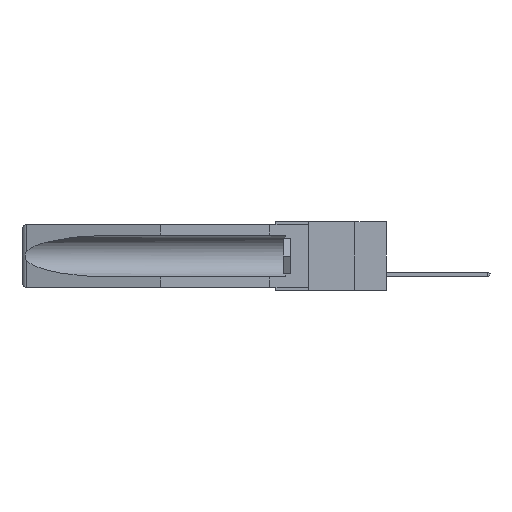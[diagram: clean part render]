
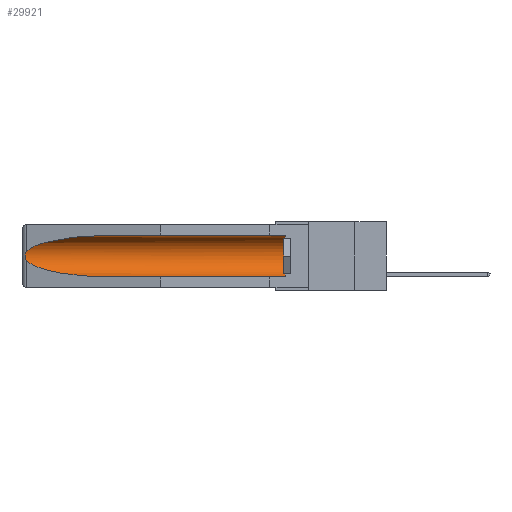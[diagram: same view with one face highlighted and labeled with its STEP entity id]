
A CAD part, left-side view. The second image highlights one B-rep face of the part: STEP entity #29921.
In plain terms, the highlighted cylindrical face has radius 2.857 mm (diameter 5.715 mm), a partial arc.
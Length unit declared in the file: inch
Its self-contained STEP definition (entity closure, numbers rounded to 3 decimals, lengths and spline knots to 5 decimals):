
#278 = EDGE_CURVE ( 'NONE', #11453, #24854, #19707, .T. ) ;
#771 = DIRECTION ( 'NONE',  ( 0., 0., 1. ) ) ;
#850 = CIRCLE ( 'NONE', #26483, 0.1125 ) ;
#1645 = VECTOR ( 'NONE', #17413, 39.37008 ) ;
#2720 = ORIENTED_EDGE ( 'NONE', *, *, #6844, .F. ) ;
#3083 = DIRECTION ( 'NONE',  ( 0., 1., 0. ) ) ;
#3252 = VERTEX_POINT ( 'NONE', #25506 ) ;
#3462 = ORIENTED_EDGE ( 'NONE', *, *, #23596, .T. ) ;
#3466 = CARTESIAN_POINT ( 'NONE',  ( 0.26537, 1.52718, -0.19328 ) ) ;
#4038 = CARTESIAN_POINT ( 'NONE',  ( 0.26597, 1.52961, -0.15275 ) ) ;
#6283 = CARTESIAN_POINT ( 'NONE',  ( 0.26537, 1.52718, -0.14972 ) ) ;
#6343 = ORIENTED_EDGE ( 'NONE', *, *, #21340, .T. ) ;
#6844 = EDGE_CURVE ( 'NONE', #32537, #19119, #28344, .T. ) ;
#7415 = CARTESIAN_POINT ( 'NONE',  ( 0.26654, 1.53092, -0.15636 ) ) ;
#8424 = ORIENTED_EDGE ( 'NONE', *, *, #31454, .T. ) ;
#8873 = CARTESIAN_POINT ( 'NONE',  ( 0.21114, 1.30732, -0.284 ) ) ;
#8904 = B_SPLINE_CURVE_WITH_KNOTS ( 'NONE', 3,
 ( #14223, #4038, #7415, #9836, #14652, #14762, #9950, #12478, #20030, #25083 ),
 .UNSPECIFIED., .F., .F.,
 ( 4, 2, 2, 2, 4 ),
 ( 0., 0.00029, 0.00058, 0.00087, 0.00117 ),
 .UNSPECIFIED. ) ;
#9836 = CARTESIAN_POINT ( 'NONE',  ( 0.2673, 1.5327, -0.16383 ) ) ;
#9950 = CARTESIAN_POINT ( 'NONE',  ( 0.2673, 1.53269, -0.17917 ) ) ;
#10229 = EDGE_CURVE ( 'NONE', #3252, #24516, #8904, .T. ) ;
#11239 = DIRECTION ( 'NONE',  ( 0., 0., 1. ) ) ;
#11369 = CARTESIAN_POINT ( 'NONE',  ( 0.155, 1.07973, -0.059 ) ) ;
#11453 = VERTEX_POINT ( 'NONE', #28151 ) ;
#12120 = ORIENTED_EDGE ( 'NONE', *, *, #278, .T. ) ;
#12140 = CARTESIAN_POINT ( 'NONE',  ( 0.155, 1.07973, -0.284 ) ) ;
#12478 = CARTESIAN_POINT ( 'NONE',  ( 0.26655, 1.53094, -0.18657 ) ) ;
#12953 = CARTESIAN_POINT ( 'NONE',  ( 0.155, -0.30754, -0.284 ) ) ;
#14223 = CARTESIAN_POINT ( 'NONE',  ( 0.26537, 1.52718, -0.14972 ) ) ;
#14652 = CARTESIAN_POINT ( 'NONE',  ( 0.2675, 1.53308, -0.16763 ) ) ;
#14762 = CARTESIAN_POINT ( 'NONE',  ( 0.2675, 1.53308, -0.17534 ) ) ;
#15697 = FACE_OUTER_BOUND ( 'NONE', #31445, .T. ) ;
#16087 = CYLINDRICAL_SURFACE ( 'NONE', #19623, 0.1125 ) ;
#16159 = CARTESIAN_POINT ( 'NONE',  ( 0.21114, 1.30732, -0.059 ) ) ;
#17135 =( BOUNDED_CURVE ( )  B_SPLINE_CURVE ( 3, ( #11369, #16159, #18687, #6283 ),
 .UNSPECIFIED., .F., .F. ) 
 B_SPLINE_CURVE_WITH_KNOTS ( ( 4, 4 ),
 ( 4.71239, 6.08839 ),
 .UNSPECIFIED. ) 
 CURVE ( )  GEOMETRIC_REPRESENTATION_ITEM ( )  RATIONAL_B_SPLINE_CURVE ( ( 1., 0.848, 0.848, 1. ) ) 
 REPRESENTATION_ITEM ( '' )  );
#17413 = DIRECTION ( 'NONE',  ( 0., 1., 0. ) ) ;
#18238 = ORIENTED_EDGE ( 'NONE', *, *, #10229, .T. ) ;
#18662 = CARTESIAN_POINT ( 'NONE',  ( 0.155, 0.126, -0.1715 ) ) ;
#18687 = CARTESIAN_POINT ( 'NONE',  ( 0.25451, 1.48313, -0.09465 ) ) ;
#19119 = VERTEX_POINT ( 'NONE', #12140 ) ;
#19623 = AXIS2_PLACEMENT_3D ( 'NONE', #30909, #3083, #771 ) ;
#19707 = LINE ( 'NONE', #29773, #1645 ) ;
#20030 = CARTESIAN_POINT ( 'NONE',  ( 0.26597, 1.5296, -0.19026 ) ) ;
#21156 = CARTESIAN_POINT ( 'NONE',  ( 0.25451, 1.48313, -0.24835 ) ) ;
#21340 = EDGE_CURVE ( 'NONE', #24854, #3252, #17135, .T. ) ;
#21830 = CARTESIAN_POINT ( 'NONE',  ( 0.155, 0.126, -0.284 ) ) ;
#23052 = DIRECTION ( 'NONE',  ( 0., 1., 0. ) ) ;
#23192 = CARTESIAN_POINT ( 'NONE',  ( 0.155, 1.07973, -0.059 ) ) ;
#23576 = VECTOR ( 'NONE', #23052, 39.37008 ) ;
#23596 = EDGE_CURVE ( 'NONE', #32537, #11453, #850, .T. ) ;
#23724 = DIRECTION ( 'NONE',  ( 0., -1., 0. ) ) ;
#24516 = VERTEX_POINT ( 'NONE', #3466 ) ;
#24854 = VERTEX_POINT ( 'NONE', #23192 ) ;
#25083 = CARTESIAN_POINT ( 'NONE',  ( 0.26537, 1.52718, -0.19328 ) ) ;
#25506 = CARTESIAN_POINT ( 'NONE',  ( 0.26537, 1.52718, -0.14972 ) ) ;
#26116 = CARTESIAN_POINT ( 'NONE',  ( 0.155, 1.07973, -0.284 ) ) ;
#26337 = CARTESIAN_POINT ( 'NONE',  ( 0.26537, 1.52718, -0.19328 ) ) ;
#26483 = AXIS2_PLACEMENT_3D ( 'NONE', #18662, #23724, #11239 ) ;
#28151 = CARTESIAN_POINT ( 'NONE',  ( 0.155, 0.126, -0.059 ) ) ;
#28344 = LINE ( 'NONE', #12953, #23576 ) ;
#28860 =( BOUNDED_CURVE ( )  B_SPLINE_CURVE ( 3, ( #26337, #21156, #8873, #26116 ),
 .UNSPECIFIED., .F., .F. ) 
 B_SPLINE_CURVE_WITH_KNOTS ( ( 4, 4 ),
 ( 0.1948, 1.5708 ),
 .UNSPECIFIED. ) 
 CURVE ( )  GEOMETRIC_REPRESENTATION_ITEM ( )  RATIONAL_B_SPLINE_CURVE ( ( 1., 0.848, 0.848, 1. ) ) 
 REPRESENTATION_ITEM ( '' )  );
#29773 = CARTESIAN_POINT ( 'NONE',  ( 0.155, -0.30754, -0.059 ) ) ;
#29921 = ADVANCED_FACE ( 'NONE', ( #15697 ), #16087, .F. ) ;
#30909 = CARTESIAN_POINT ( 'NONE',  ( 0.155, -0.30754, -0.1715 ) ) ;
#31445 = EDGE_LOOP ( 'NONE', ( #6343, #18238, #8424, #2720, #3462, #12120 ) ) ;
#31454 = EDGE_CURVE ( 'NONE', #24516, #19119, #28860, .T. ) ;
#32537 = VERTEX_POINT ( 'NONE', #21830 ) ;
